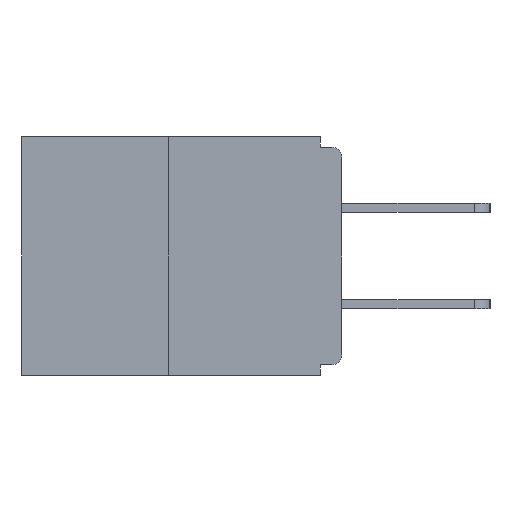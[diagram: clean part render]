
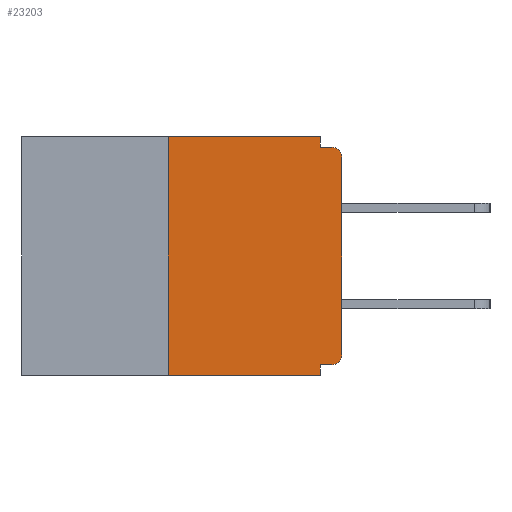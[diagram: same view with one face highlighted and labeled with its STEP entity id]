
A CAD part, left-side view. The second image highlights one B-rep face of the part: STEP entity #23203.
In plain terms, the highlighted planar face has unit normal (-1, 0, 0).
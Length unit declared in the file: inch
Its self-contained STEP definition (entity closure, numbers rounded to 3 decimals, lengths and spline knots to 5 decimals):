
#153 = CARTESIAN_POINT ( 'NONE',  ( 0., 0.25, -0.343 ) ) ;
#223 = PLANE ( 'NONE',  #3415 ) ;
#696 = VECTOR ( 'NONE', #7246, 39.37008 ) ;
#1325 = DIRECTION ( 'NONE',  ( 0., -1., 0. ) ) ;
#1359 = AXIS2_PLACEMENT_3D ( 'NONE', #14290, #5186, #14408 ) ;
#1445 = VERTEX_POINT ( 'NONE', #22843 ) ;
#2242 = CIRCLE ( 'NONE', #8315, 0.015 ) ;
#2368 = CARTESIAN_POINT ( 'NONE',  ( 0., 0.46, 0. ) ) ;
#2411 = EDGE_CURVE ( 'NONE', #23476, #16988, #21538, .T. ) ;
#2415 = CARTESIAN_POINT ( 'NONE',  ( 0., 0., -0.328 ) ) ;
#2418 = LINE ( 'NONE', #19032, #8197 ) ;
#3120 = CARTESIAN_POINT ( 'NONE',  ( 0., 0.46, -0.343 ) ) ;
#3415 = AXIS2_PLACEMENT_3D ( 'NONE', #14795, #18278, #13004 ) ;
#3528 = LINE ( 'NONE', #10811, #5291 ) ;
#4067 = DIRECTION ( 'NONE',  ( 0., 0., -1. ) ) ;
#4832 = CARTESIAN_POINT ( 'NONE',  ( 0., 0.031, -0.015 ) ) ;
#5186 = DIRECTION ( 'NONE',  ( -1., 0., 0. ) ) ;
#5291 = VECTOR ( 'NONE', #18375, 39.37008 ) ;
#5793 = ORIENTED_EDGE ( 'NONE', *, *, #22026, .F. ) ;
#6916 = VECTOR ( 'NONE', #20494, 39.37008 ) ;
#7000 = ORIENTED_EDGE ( 'NONE', *, *, #7648, .F. ) ;
#7246 = DIRECTION ( 'NONE',  ( 0., 0., 1. ) ) ;
#7648 = EDGE_CURVE ( 'NONE', #22982, #1445, #2418, .T. ) ;
#8139 = CARTESIAN_POINT ( 'NONE',  ( 0., 0.031, 0. ) ) ;
#8197 = VECTOR ( 'NONE', #4067, 39.37008 ) ;
#8315 = AXIS2_PLACEMENT_3D ( 'NONE', #15861, #23204, #14048 ) ;
#9329 = VERTEX_POINT ( 'NONE', #4832 ) ;
#9333 = CARTESIAN_POINT ( 'NONE',  ( 0., 0.015, -0.328 ) ) ;
#9479 = EDGE_CURVE ( 'NONE', #18805, #20124, #11661, .T. ) ;
#9483 = CARTESIAN_POINT ( 'NONE',  ( 0., 0.25, 0. ) ) ;
#9634 = LINE ( 'NONE', #11446, #22146 ) ;
#9751 = DIRECTION ( 'NONE',  ( 0., 0., -1. ) ) ;
#9897 = VERTEX_POINT ( 'NONE', #9333 ) ;
#10206 = DIRECTION ( 'NONE',  ( 0., 0., 1. ) ) ;
#10410 = ORIENTED_EDGE ( 'NONE', *, *, #2411, .F. ) ;
#10413 = ORIENTED_EDGE ( 'NONE', *, *, #20528, .T. ) ;
#10708 = EDGE_CURVE ( 'NONE', #9329, #20124, #3528, .T. ) ;
#10811 = CARTESIAN_POINT ( 'NONE',  ( 0., 0., -0.015 ) ) ;
#11417 = ORIENTED_EDGE ( 'NONE', *, *, #9479, .T. ) ;
#11446 = CARTESIAN_POINT ( 'NONE',  ( 0., 0.031, 0. ) ) ;
#11661 = CIRCLE ( 'NONE', #1359, 0.015 ) ;
#12138 = VECTOR ( 'NONE', #10206, 39.37008 ) ;
#12247 = VERTEX_POINT ( 'NONE', #8139 ) ;
#12264 = ORIENTED_EDGE ( 'NONE', *, *, #13934, .F. ) ;
#12778 = CARTESIAN_POINT ( 'NONE',  ( 0., 0., -0.313 ) ) ;
#13004 = DIRECTION ( 'NONE',  ( 0., 0., -1. ) ) ;
#13243 = EDGE_CURVE ( 'NONE', #9897, #22982, #22671, .T. ) ;
#13373 = EDGE_CURVE ( 'NONE', #23476, #1445, #23386, .T. ) ;
#13934 = EDGE_CURVE ( 'NONE', #16988, #12247, #18749, .T. ) ;
#14048 = DIRECTION ( 'NONE',  ( 0., 0., -1. ) ) ;
#14137 = ORIENTED_EDGE ( 'NONE', *, *, #13373, .T. ) ;
#14290 = CARTESIAN_POINT ( 'NONE',  ( 0., 0.015, -0.03 ) ) ;
#14408 = DIRECTION ( 'NONE',  ( 0., 0., -1. ) ) ;
#14552 = CARTESIAN_POINT ( 'NONE',  ( 0., 0.25, 0. ) ) ;
#14795 = CARTESIAN_POINT ( 'NONE',  ( 0., 0.46, 0. ) ) ;
#15350 = VECTOR ( 'NONE', #17072, 39.37008 ) ;
#15861 = CARTESIAN_POINT ( 'NONE',  ( 0., 0.015, -0.313 ) ) ;
#16988 = VERTEX_POINT ( 'NONE', #9483 ) ;
#17072 = DIRECTION ( 'NONE',  ( 0., -1., 0. ) ) ;
#17302 = LINE ( 'NONE', #19211, #12138 ) ;
#17697 = CARTESIAN_POINT ( 'NONE',  ( 0., 0.031, -0.328 ) ) ;
#18278 = DIRECTION ( 'NONE',  ( 1., 0., 0. ) ) ;
#18375 = DIRECTION ( 'NONE',  ( 0., -1., 0. ) ) ;
#18749 = LINE ( 'NONE', #2368, #15350 ) ;
#18805 = VERTEX_POINT ( 'NONE', #21167 ) ;
#19032 = CARTESIAN_POINT ( 'NONE',  ( 0., 0.031, -0.343 ) ) ;
#19104 = ORIENTED_EDGE ( 'NONE', *, *, #13243, .F. ) ;
#19211 = CARTESIAN_POINT ( 'NONE',  ( 0., 0., 0. ) ) ;
#19284 = EDGE_LOOP ( 'NONE', ( #12264, #10410, #14137, #7000, #19104, #21946, #10413, #11417, #21227, #5793 ) ) ;
#19544 = VECTOR ( 'NONE', #1325, 39.37008 ) ;
#19854 = VERTEX_POINT ( 'NONE', #12778 ) ;
#20124 = VERTEX_POINT ( 'NONE', #21540 ) ;
#20444 = FACE_OUTER_BOUND ( 'NONE', #19284, .T. ) ;
#20494 = DIRECTION ( 'NONE',  ( 0., 1., 0. ) ) ;
#20528 = EDGE_CURVE ( 'NONE', #19854, #18805, #17302, .T. ) ;
#20547 = EDGE_CURVE ( 'NONE', #9897, #19854, #2242, .T. ) ;
#21167 = CARTESIAN_POINT ( 'NONE',  ( 0., 0., -0.03 ) ) ;
#21227 = ORIENTED_EDGE ( 'NONE', *, *, #10708, .F. ) ;
#21538 = LINE ( 'NONE', #14552, #696 ) ;
#21540 = CARTESIAN_POINT ( 'NONE',  ( 0., 0.015, -0.015 ) ) ;
#21946 = ORIENTED_EDGE ( 'NONE', *, *, #20547, .T. ) ;
#22026 = EDGE_CURVE ( 'NONE', #12247, #9329, #9634, .T. ) ;
#22146 = VECTOR ( 'NONE', #9751, 39.37008 ) ;
#22671 = LINE ( 'NONE', #2415, #6916 ) ;
#22843 = CARTESIAN_POINT ( 'NONE',  ( 0., 0.031, -0.343 ) ) ;
#22982 = VERTEX_POINT ( 'NONE', #17697 ) ;
#23203 = ADVANCED_FACE ( 'NONE', ( #20444 ), #223, .F. ) ;
#23204 = DIRECTION ( 'NONE',  ( -1., 0., 0. ) ) ;
#23386 = LINE ( 'NONE', #3120, #19544 ) ;
#23476 = VERTEX_POINT ( 'NONE', #153 ) ;
